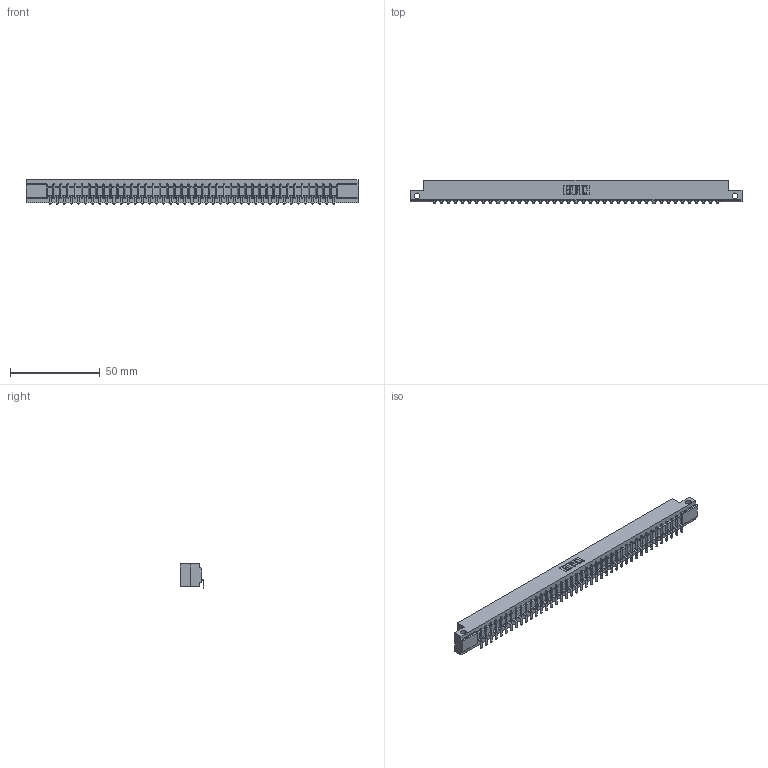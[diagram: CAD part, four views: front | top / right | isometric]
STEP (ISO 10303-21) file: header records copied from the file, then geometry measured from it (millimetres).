
FILE_DESCRIPTION (( 'STEP AP203' ), '1' );
FILE_NAME ('357-041-553-112.STEP', '2019-09-17T09:50:03', ( '' ), ( '' ), 'SwSTEP 2.0', 'SolidWorks 2016', '' );
FILE_SCHEMA (( 'CONFIG_CONTROL_DESIGN' ));
Length unit declared in the file: inch
Products named in the file (3): 357-041-553-112; 307 Part_.128 Dia Side Mounting Holes; 307-290-002_553
Assembly tree (42 placements, depth 2):
  357-041-553-112
    307 Part_.128 Dia Side Mounting Holes
    307-290-002_553  x41
Bounding box: 185.47 x 13.32 x 13.5 mm (x, y, z)
Volume: 19698 mm3; surface area: 24727.7 mm2
Topology: 42 solids, 42 shells, 3358 faces, 10327 edges, 6770 vertices
Faces by surface type: plane 1997, cylinder 1277, sphere 84
Entity records: 36128 total; most frequent: CARTESIAN_POINT 6096, ORIENTED_EDGE 6086, DIRECTION 5923, EDGE_CURVE 3043, LINE 2329, VECTOR 2329, VERTEX_POINT 1970, AXIS2_PLACEMENT_3D 1797
